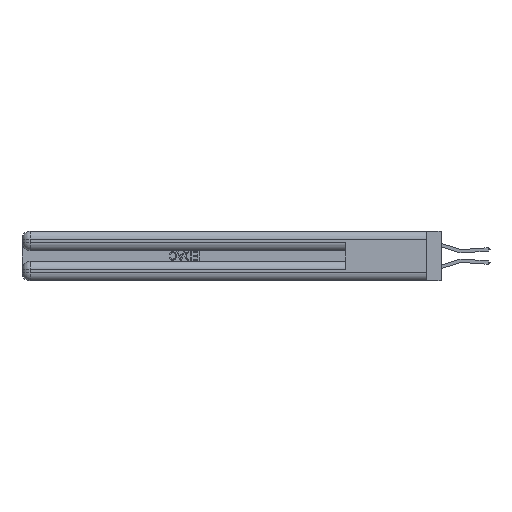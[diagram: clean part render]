
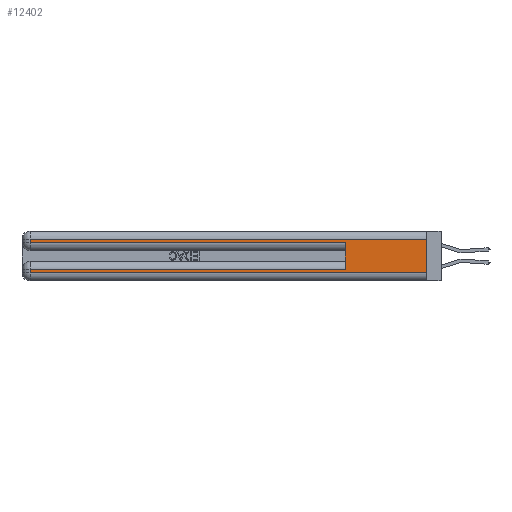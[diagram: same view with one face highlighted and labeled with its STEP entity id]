
A CAD part, left-side view. The second image highlights one B-rep face of the part: STEP entity #12402.
In plain terms, the highlighted planar face has unit normal (-1, 0, 0).
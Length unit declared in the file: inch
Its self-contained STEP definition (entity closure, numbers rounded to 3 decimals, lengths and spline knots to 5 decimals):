
#479 = DIRECTION ( 'NONE',  ( 1., 0., 0. ) ) ;
#2969 = DIRECTION ( 'NONE',  ( 0., 0., 1. ) ) ;
#3104 = DIRECTION ( 'NONE',  ( 0., 0., -1. ) ) ;
#3459 = CARTESIAN_POINT ( 'NONE',  ( 0., 2.94, 0.06 ) ) ;
#3467 = CARTESIAN_POINT ( 'NONE',  ( 0., 0.6, 0.145 ) ) ;
#3496 = VERTEX_POINT ( 'NONE', #15536 ) ;
#4068 = LINE ( 'NONE', #8089, #35898 ) ;
#5346 = ORIENTED_EDGE ( 'NONE', *, *, #10788, .F. ) ;
#5871 = VERTEX_POINT ( 'NONE', #32394 ) ;
#6162 = VECTOR ( 'NONE', #21172, 39.37008 ) ;
#6988 = EDGE_LOOP ( 'NONE', ( #5346, #20630, #30938, #29423, #16945, #47579, #8646, #37956 ) ) ;
#7855 = LINE ( 'NONE', #32933, #46736 ) ;
#8089 = CARTESIAN_POINT ( 'NONE',  ( 0., 0., 0.06 ) ) ;
#8120 = DIRECTION ( 'NONE',  ( 0., 0., -1. ) ) ;
#8646 = ORIENTED_EDGE ( 'NONE', *, *, #8670, .T. ) ;
#8670 = EDGE_CURVE ( 'NONE', #25282, #12988, #36206, .T. ) ;
#8768 = CARTESIAN_POINT ( 'NONE',  ( 0., 0.6, 0.085 ) ) ;
#8775 = LINE ( 'NONE', #40223, #26461 ) ;
#9277 = EDGE_CURVE ( 'NONE', #12594, #5871, #42000, .T. ) ;
#9416 = VECTOR ( 'NONE', #37396, 39.37008 ) ;
#10428 = PLANE ( 'NONE',  #30576 ) ;
#10788 = EDGE_CURVE ( 'NONE', #3496, #29860, #23053, .T. ) ;
#12402 = ADVANCED_FACE ( 'NONE', ( #37143 ), #10428, .F. ) ;
#12409 = EDGE_CURVE ( 'NONE', #22563, #27008, #43590, .T. ) ;
#12594 = VERTEX_POINT ( 'NONE', #8768 ) ;
#12988 = VERTEX_POINT ( 'NONE', #3459 ) ;
#13236 = EDGE_CURVE ( 'NONE', #12988, #29860, #4068, .T. ) ;
#15536 = CARTESIAN_POINT ( 'NONE',  ( 0., 0., 0.31 ) ) ;
#16444 = CARTESIAN_POINT ( 'NONE',  ( 0., 2.94, 0.085 ) ) ;
#16945 = ORIENTED_EDGE ( 'NONE', *, *, #9277, .F. ) ;
#20538 = CARTESIAN_POINT ( 'NONE',  ( 0., 2.94, 0.37 ) ) ;
#20630 = ORIENTED_EDGE ( 'NONE', *, *, #34769, .T. ) ;
#21172 = DIRECTION ( 'NONE',  ( 0., 0., -1. ) ) ;
#21965 = CARTESIAN_POINT ( 'NONE',  ( 0., 2.94, 0.31 ) ) ;
#22563 = VERTEX_POINT ( 'NONE', #21965 ) ;
#22645 = CARTESIAN_POINT ( 'NONE',  ( 0., 0., 0.37 ) ) ;
#23025 = CARTESIAN_POINT ( 'NONE',  ( 0., 0., 0.06 ) ) ;
#23053 = LINE ( 'NONE', #33863, #41837 ) ;
#23125 = CARTESIAN_POINT ( 'NONE',  ( 0., 2.94, 0.285 ) ) ;
#24396 = EDGE_CURVE ( 'NONE', #12594, #25282, #7855, .T. ) ;
#25282 = VERTEX_POINT ( 'NONE', #16444 ) ;
#26132 = VECTOR ( 'NONE', #2969, 39.37008 ) ;
#26461 = VECTOR ( 'NONE', #47130, 39.37008 ) ;
#27008 = VERTEX_POINT ( 'NONE', #23125 ) ;
#27717 = LINE ( 'NONE', #29876, #9416 ) ;
#29423 = ORIENTED_EDGE ( 'NONE', *, *, #48168, .T. ) ;
#29860 = VERTEX_POINT ( 'NONE', #23025 ) ;
#29876 = CARTESIAN_POINT ( 'NONE',  ( 0., 0., 0.285 ) ) ;
#30576 = AXIS2_PLACEMENT_3D ( 'NONE', #22645, #479, #8120 ) ;
#30938 = ORIENTED_EDGE ( 'NONE', *, *, #12409, .T. ) ;
#32394 = CARTESIAN_POINT ( 'NONE',  ( 0., 0.6, 0.285 ) ) ;
#32933 = CARTESIAN_POINT ( 'NONE',  ( 0., 0., 0.085 ) ) ;
#33863 = CARTESIAN_POINT ( 'NONE',  ( 0., 0., 0.37 ) ) ;
#34769 = EDGE_CURVE ( 'NONE', #3496, #22563, #8775, .T. ) ;
#35898 = VECTOR ( 'NONE', #41994, 39.37008 ) ;
#36206 = LINE ( 'NONE', #20538, #6162 ) ;
#37143 = FACE_OUTER_BOUND ( 'NONE', #6988, .T. ) ;
#37396 = DIRECTION ( 'NONE',  ( 0., -1., 0. ) ) ;
#37809 = DIRECTION ( 'NONE',  ( 0., 0., -1. ) ) ;
#37956 = ORIENTED_EDGE ( 'NONE', *, *, #13236, .T. ) ;
#38039 = DIRECTION ( 'NONE',  ( 0., 1., 0. ) ) ;
#40223 = CARTESIAN_POINT ( 'NONE',  ( 0., 0., 0.31 ) ) ;
#41837 = VECTOR ( 'NONE', #37809, 39.37008 ) ;
#41994 = DIRECTION ( 'NONE',  ( 0., -1., 0. ) ) ;
#42000 = LINE ( 'NONE', #3467, #26132 ) ;
#42519 = CARTESIAN_POINT ( 'NONE',  ( 0., 2.94, 0.37 ) ) ;
#43590 = LINE ( 'NONE', #42519, #47682 ) ;
#46736 = VECTOR ( 'NONE', #38039, 39.37008 ) ;
#47130 = DIRECTION ( 'NONE',  ( 0., 1., 0. ) ) ;
#47579 = ORIENTED_EDGE ( 'NONE', *, *, #24396, .T. ) ;
#47682 = VECTOR ( 'NONE', #3104, 39.37008 ) ;
#48168 = EDGE_CURVE ( 'NONE', #27008, #5871, #27717, .T. ) ;
